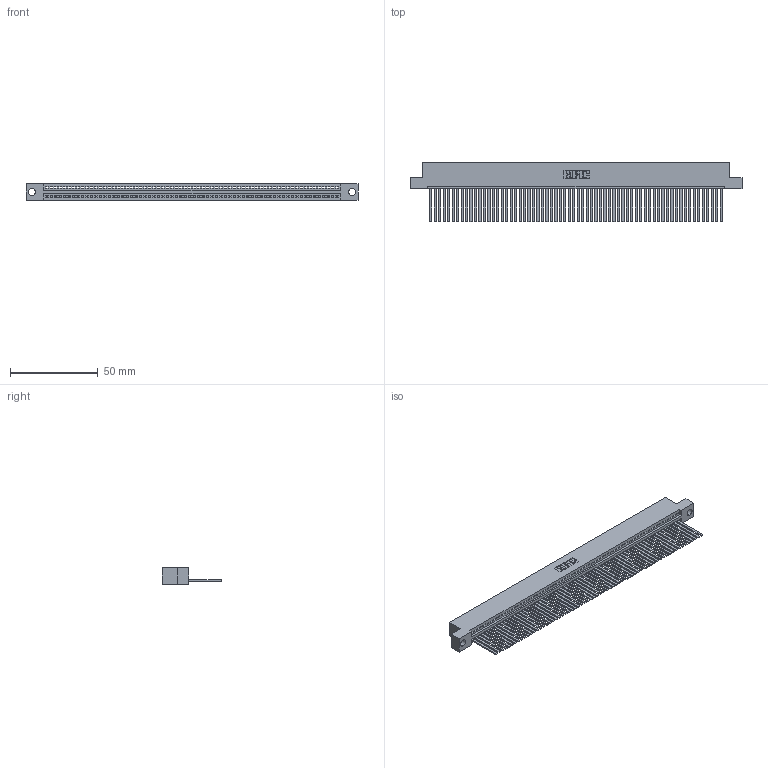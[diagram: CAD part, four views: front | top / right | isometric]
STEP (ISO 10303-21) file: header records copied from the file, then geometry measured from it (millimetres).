
FILE_DESCRIPTION (( 'STEP AP203' ), '1' );
FILE_NAME ('395-066-544-104.STEP', '2021-05-31T22:07:19', ( '' ), ( '' ), 'SwSTEP 2.0', 'SolidWorks 2020', '' );
FILE_SCHEMA (( 'CONFIG_CONTROL_DESIGN' ));
Length unit declared in the file: inch
Products named in the file (3): 345 Part_Flush Mounting Lugs - 0.156 Dia-TI; 345-292-001_345-293-144; 395-066-544-104
Assembly tree (67 placements, depth 2):
  395-066-544-104
    345 Part_Flush Mounting Lugs - 0.156 Dia-TI
    345-292-001_345-293-144  x66
Bounding box: 188.85 x 33.96 x 9.4 mm (x, y, z)
Volume: 18792.1 mm3; surface area: 27436.4 mm2
Topology: 67 solids, 67 shells, 3572 faces, 10805 edges, 7114 vertices
Faces by surface type: plane 2470, cylinder 1102
Entity records: 46677 total; most frequent: CARTESIAN_POINT 8092, ORIENTED_EDGE 8090, DIRECTION 7029, EDGE_CURVE 4045, LINE 3653, VECTOR 3653, VERTEX_POINT 2694, AXIS2_PLACEMENT_3D 1688
